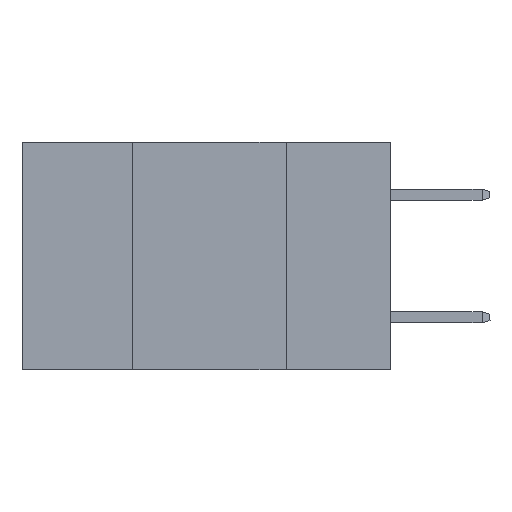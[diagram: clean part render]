
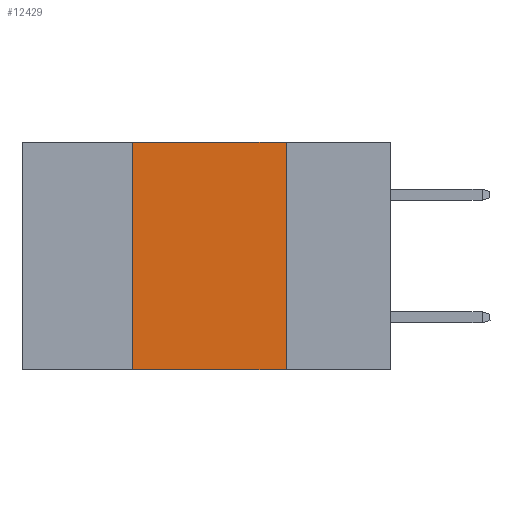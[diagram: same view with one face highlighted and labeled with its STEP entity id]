
A CAD part, left-side view. The second image highlights one B-rep face of the part: STEP entity #12429.
In plain terms, the highlighted planar face has unit normal (-1, 0, 0).
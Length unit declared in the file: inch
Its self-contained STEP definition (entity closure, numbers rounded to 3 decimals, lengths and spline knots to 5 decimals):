
#26 = LINE ( 'NONE', #9295, #10367 ) ;
#232 = CARTESIAN_POINT ( 'NONE',  ( 0., 0.6, 0. ) ) ;
#609 = LINE ( 'NONE', #8171, #10641 ) ;
#1938 = ORIENTED_EDGE ( 'NONE', *, *, #10019, .F. ) ;
#1982 = EDGE_CURVE ( 'NONE', #7400, #7618, #26, .T. ) ;
#2095 = EDGE_CURVE ( 'NONE', #7618, #5499, #6601, .T. ) ;
#2315 = PLANE ( 'NONE',  #2324 ) ;
#2324 = AXIS2_PLACEMENT_3D ( 'NONE', #232, #9304, #3387 ) ;
#3387 = DIRECTION ( 'NONE',  ( 0., 0., -1. ) ) ;
#3406 = EDGE_CURVE ( 'NONE', #7400, #3661, #609, .T. ) ;
#3661 = VERTEX_POINT ( 'NONE', #4798 ) ;
#3701 = CARTESIAN_POINT ( 'NONE',  ( 0., 0.42, 0. ) ) ;
#4390 = DIRECTION ( 'NONE',  ( 0., 0., -1. ) ) ;
#4735 = ORIENTED_EDGE ( 'NONE', *, *, #2095, .F. ) ;
#4798 = CARTESIAN_POINT ( 'NONE',  ( 0., 0.17, -0.37 ) ) ;
#5049 = ORIENTED_EDGE ( 'NONE', *, *, #3406, .T. ) ;
#5367 = CARTESIAN_POINT ( 'NONE',  ( 0., 0.17, 0. ) ) ;
#5499 = VERTEX_POINT ( 'NONE', #11782 ) ;
#6552 = DIRECTION ( 'NONE',  ( 0., -1., 0. ) ) ;
#6561 = CARTESIAN_POINT ( 'NONE',  ( 0., 0.6, 0. ) ) ;
#6601 = LINE ( 'NONE', #6561, #9178 ) ;
#6707 = EDGE_LOOP ( 'NONE', ( #1938, #4735, #7352, #5049 ) ) ;
#7352 = ORIENTED_EDGE ( 'NONE', *, *, #1982, .F. ) ;
#7373 = CARTESIAN_POINT ( 'NONE',  ( 0., 0.42, -0.37 ) ) ;
#7400 = VERTEX_POINT ( 'NONE', #7373 ) ;
#7404 = FACE_OUTER_BOUND ( 'NONE', #6707, .T. ) ;
#7503 = DIRECTION ( 'NONE',  ( 0., -1., 0. ) ) ;
#7618 = VERTEX_POINT ( 'NONE', #3701 ) ;
#7633 = VECTOR ( 'NONE', #4390, 39.37008 ) ;
#8171 = CARTESIAN_POINT ( 'NONE',  ( 0., 0.6, -0.37 ) ) ;
#9178 = VECTOR ( 'NONE', #6552, 39.37008 ) ;
#9295 = CARTESIAN_POINT ( 'NONE',  ( 0., 0.42, 0. ) ) ;
#9304 = DIRECTION ( 'NONE',  ( 1., 0., 0. ) ) ;
#10019 = EDGE_CURVE ( 'NONE', #5499, #3661, #10477, .T. ) ;
#10367 = VECTOR ( 'NONE', #10416, 39.37008 ) ;
#10416 = DIRECTION ( 'NONE',  ( 0., 0., 1. ) ) ;
#10477 = LINE ( 'NONE', #5367, #7633 ) ;
#10641 = VECTOR ( 'NONE', #7503, 39.37008 ) ;
#11782 = CARTESIAN_POINT ( 'NONE',  ( 0., 0.17, 0. ) ) ;
#12429 = ADVANCED_FACE ( 'NONE', ( #7404 ), #2315, .F. ) ;
